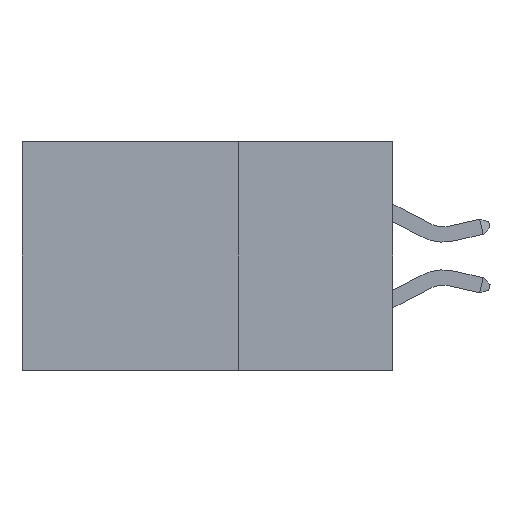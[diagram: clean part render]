
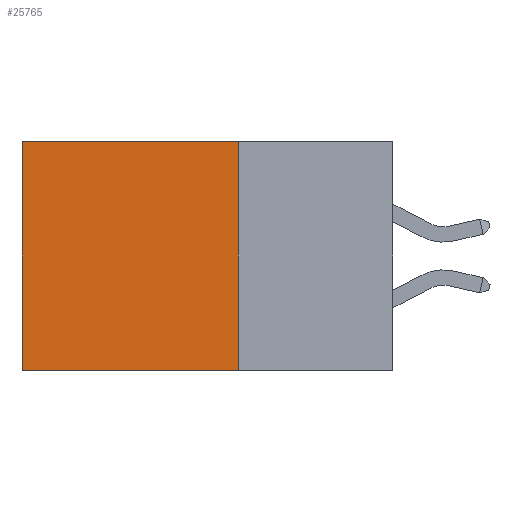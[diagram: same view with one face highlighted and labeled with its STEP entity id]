
A CAD part, left-side view. The second image highlights one B-rep face of the part: STEP entity #25765.
In plain terms, the highlighted planar face has unit normal (-1, 0, 0).
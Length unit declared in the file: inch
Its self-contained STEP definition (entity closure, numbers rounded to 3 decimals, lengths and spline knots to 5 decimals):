
#352 = PLANE ( 'NONE',  #15297 ) ;
#544 = FACE_OUTER_BOUND ( 'NONE', #6969, .T. ) ;
#834 = VERTEX_POINT ( 'NONE', #7770 ) ;
#1464 = EDGE_CURVE ( 'NONE', #834, #11982, #5004, .T. ) ;
#1496 = CARTESIAN_POINT ( 'NONE',  ( 0.2875, 0.6, -0.37 ) ) ;
#1997 = CARTESIAN_POINT ( 'NONE',  ( 0.2875, 0.6, 0. ) ) ;
#2624 = CARTESIAN_POINT ( 'NONE',  ( 0.2875, 0.25, -0.37 ) ) ;
#2762 = CARTESIAN_POINT ( 'NONE',  ( 0.2875, 0.25, 0. ) ) ;
#4765 = DIRECTION ( 'NONE',  ( 1., 0., 0. ) ) ;
#4867 = ORIENTED_EDGE ( 'NONE', *, *, #10218, .F. ) ;
#4973 = ORIENTED_EDGE ( 'NONE', *, *, #1464, .T. ) ;
#5004 = LINE ( 'NONE', #24092, #8093 ) ;
#5253 = ORIENTED_EDGE ( 'NONE', *, *, #8169, .T. ) ;
#6032 = DIRECTION ( 'NONE',  ( 0., 1., 0. ) ) ;
#6596 = VECTOR ( 'NONE', #8054, 39.37008 ) ;
#6969 = EDGE_LOOP ( 'NONE', ( #5253, #4867, #7689, #4973 ) ) ;
#7689 = ORIENTED_EDGE ( 'NONE', *, *, #12823, .F. ) ;
#7770 = CARTESIAN_POINT ( 'NONE',  ( 0.2875, 0.25, 0. ) ) ;
#8054 = DIRECTION ( 'NONE',  ( 0., 0., -1. ) ) ;
#8093 = VECTOR ( 'NONE', #19970, 39.37008 ) ;
#8169 = EDGE_CURVE ( 'NONE', #11982, #17887, #11974, .T. ) ;
#8537 = LINE ( 'NONE', #18434, #23954 ) ;
#10218 = EDGE_CURVE ( 'NONE', #17718, #17887, #23486, .T. ) ;
#10347 = DIRECTION ( 'NONE',  ( 0., 0., -1. ) ) ;
#11974 = LINE ( 'NONE', #1997, #6596 ) ;
#11982 = VERTEX_POINT ( 'NONE', #15073 ) ;
#12823 = EDGE_CURVE ( 'NONE', #834, #17718, #8537, .T. ) ;
#15073 = CARTESIAN_POINT ( 'NONE',  ( 0.2875, 0.6, 0. ) ) ;
#15297 = AXIS2_PLACEMENT_3D ( 'NONE', #2762, #4765, #10347 ) ;
#17718 = VERTEX_POINT ( 'NONE', #23776 ) ;
#17887 = VERTEX_POINT ( 'NONE', #1496 ) ;
#18138 = VECTOR ( 'NONE', #6032, 39.37008 ) ;
#18434 = CARTESIAN_POINT ( 'NONE',  ( 0.2875, 0.25, 0. ) ) ;
#19970 = DIRECTION ( 'NONE',  ( 0., 1., 0. ) ) ;
#23486 = LINE ( 'NONE', #2624, #18138 ) ;
#23776 = CARTESIAN_POINT ( 'NONE',  ( 0.2875, 0.25, -0.37 ) ) ;
#23954 = VECTOR ( 'NONE', #24498, 39.37008 ) ;
#24092 = CARTESIAN_POINT ( 'NONE',  ( 0.2875, 0.25, 0. ) ) ;
#24498 = DIRECTION ( 'NONE',  ( 0., 0., -1. ) ) ;
#25765 = ADVANCED_FACE ( 'NONE', ( #544 ), #352, .F. ) ;
